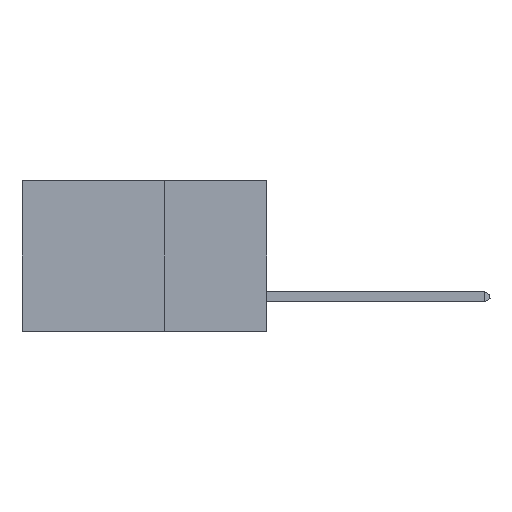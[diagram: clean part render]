
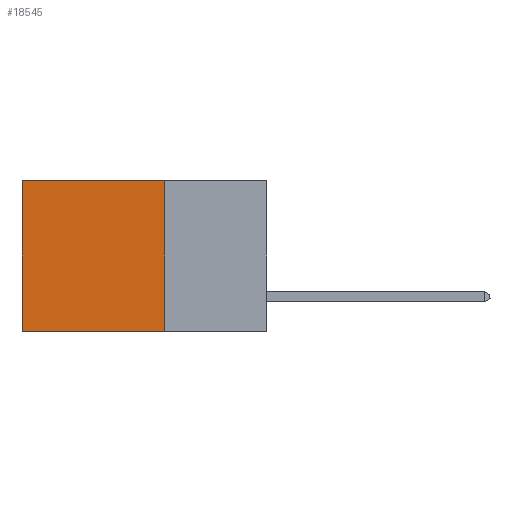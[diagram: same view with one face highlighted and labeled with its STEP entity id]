
A CAD part, left-side view. The second image highlights one B-rep face of the part: STEP entity #18545.
In plain terms, the highlighted planar face has unit normal (-1, 0, 0).
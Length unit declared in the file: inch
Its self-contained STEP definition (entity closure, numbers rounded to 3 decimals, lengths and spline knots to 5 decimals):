
#107 = EDGE_CURVE ( 'NONE', #4959, #17439, #7801, .T. ) ;
#485 = EDGE_CURVE ( 'NONE', #4568, #4775, #15406, .T. ) ;
#666 = CARTESIAN_POINT ( 'NONE',  ( 0.2875, 0.25, 0. ) ) ;
#1821 = LINE ( 'NONE', #5456, #23093 ) ;
#2605 = VECTOR ( 'NONE', #20310, 39.37008 ) ;
#4489 = VECTOR ( 'NONE', #29896, 39.37008 ) ;
#4568 = VERTEX_POINT ( 'NONE', #24927 ) ;
#4775 = VERTEX_POINT ( 'NONE', #13158 ) ;
#4959 = VERTEX_POINT ( 'NONE', #14215 ) ;
#5456 = CARTESIAN_POINT ( 'NONE',  ( 0.2875, 0.25, -0.37 ) ) ;
#6491 = ORIENTED_EDGE ( 'NONE', *, *, #107, .F. ) ;
#6808 = CARTESIAN_POINT ( 'NONE',  ( 0.2875, 0.25, 0. ) ) ;
#6913 = DIRECTION ( 'NONE',  ( 1., 0., 0. ) ) ;
#7109 = DIRECTION ( 'NONE',  ( 0., 0., -1. ) ) ;
#7801 = LINE ( 'NONE', #6808, #4489 ) ;
#8832 = CARTESIAN_POINT ( 'NONE',  ( 0.2875, 0.6, 0. ) ) ;
#10009 = DIRECTION ( 'NONE',  ( 0., 1., 0. ) ) ;
#10015 = AXIS2_PLACEMENT_3D ( 'NONE', #20746, #6913, #7109 ) ;
#10210 = CARTESIAN_POINT ( 'NONE',  ( 0.2875, 0.25, -0.37 ) ) ;
#10718 = EDGE_CURVE ( 'NONE', #17439, #4775, #1821, .T. ) ;
#11631 = ORIENTED_EDGE ( 'NONE', *, *, #18066, .T. ) ;
#13158 = CARTESIAN_POINT ( 'NONE',  ( 0.2875, 0.6, -0.37 ) ) ;
#13570 = LINE ( 'NONE', #666, #24939 ) ;
#14215 = CARTESIAN_POINT ( 'NONE',  ( 0.2875, 0.25, 0. ) ) ;
#14971 = ORIENTED_EDGE ( 'NONE', *, *, #485, .T. ) ;
#15303 = FACE_OUTER_BOUND ( 'NONE', #20060, .T. ) ;
#15406 = LINE ( 'NONE', #8832, #2605 ) ;
#17242 = ORIENTED_EDGE ( 'NONE', *, *, #10718, .F. ) ;
#17439 = VERTEX_POINT ( 'NONE', #10210 ) ;
#18066 = EDGE_CURVE ( 'NONE', #4959, #4568, #13570, .T. ) ;
#18545 = ADVANCED_FACE ( 'NONE', ( #15303 ), #25511, .F. ) ;
#20060 = EDGE_LOOP ( 'NONE', ( #14971, #17242, #6491, #11631 ) ) ;
#20310 = DIRECTION ( 'NONE',  ( 0., 0., -1. ) ) ;
#20746 = CARTESIAN_POINT ( 'NONE',  ( 0.2875, 0.25, 0. ) ) ;
#23093 = VECTOR ( 'NONE', #26562, 39.37008 ) ;
#24927 = CARTESIAN_POINT ( 'NONE',  ( 0.2875, 0.6, 0. ) ) ;
#24939 = VECTOR ( 'NONE', #10009, 39.37008 ) ;
#25511 = PLANE ( 'NONE',  #10015 ) ;
#26562 = DIRECTION ( 'NONE',  ( 0., 1., 0. ) ) ;
#29896 = DIRECTION ( 'NONE',  ( 0., 0., -1. ) ) ;
